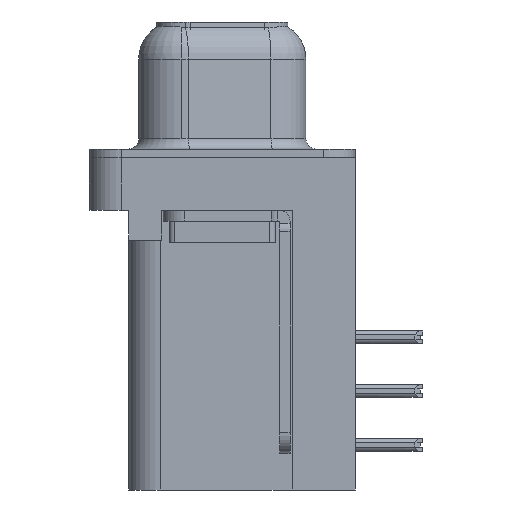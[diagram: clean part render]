
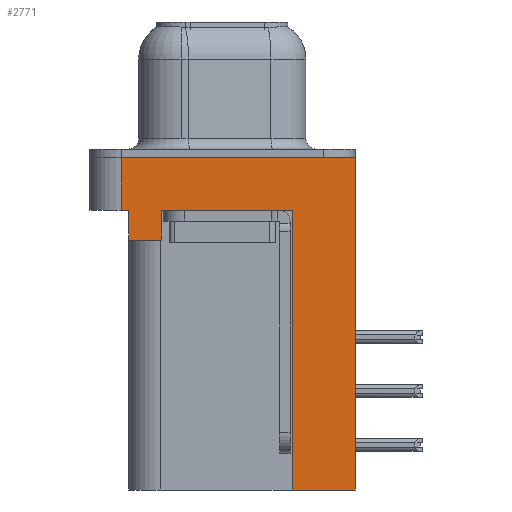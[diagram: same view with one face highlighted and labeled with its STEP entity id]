
A CAD part, left-side view. The second image highlights one B-rep face of the part: STEP entity #2771.
In plain terms, the highlighted planar face has unit normal (-1, 0, 0).
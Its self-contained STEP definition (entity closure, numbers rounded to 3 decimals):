
#1096 = EDGE_CURVE ( 'NONE', #31245, #6564, #27207, .T. ) ;
#1866 = LINE ( 'NONE', #28821, #1961 ) ;
#1961 = VECTOR ( 'NONE', #20287, 1000. ) ;
#2158 = FACE_OUTER_BOUND ( 'NONE', #15014, .T. ) ;
#2771 = ADVANCED_FACE ( 'NONE', ( #2158 ), #19928, .T. ) ;
#3632 = VERTEX_POINT ( 'NONE', #32610 ) ;
#3894 = CARTESIAN_POINT ( 'NONE',  ( -2.935, -6.275, 0. ) ) ;
#6511 = VERTEX_POINT ( 'NONE', #27391 ) ;
#6564 = VERTEX_POINT ( 'NONE', #19073 ) ;
#6860 = VERTEX_POINT ( 'NONE', #9799 ) ;
#7109 = DIRECTION ( 'NONE',  ( 0., 0., 1. ) ) ;
#7168 = ORIENTED_EDGE ( 'NONE', *, *, #12421, .T. ) ;
#7468 = DIRECTION ( 'NONE',  ( 0., -1., 0. ) ) ;
#7547 = VERTEX_POINT ( 'NONE', #25206 ) ;
#8187 = EDGE_CURVE ( 'NONE', #27792, #27473, #30651, .T. ) ;
#9799 = CARTESIAN_POINT ( 'NONE',  ( -2.935, 2.895, -2.5 ) ) ;
#10481 = VECTOR ( 'NONE', #7468, 1000. ) ;
#10658 = CARTESIAN_POINT ( 'NONE',  ( -2.935, 4.775, -2.5 ) ) ;
#10858 = LINE ( 'NONE', #24456, #10481 ) ;
#12023 = CARTESIAN_POINT ( 'NONE',  ( -2.935, 4.425, -3.9 ) ) ;
#12200 = AXIS2_PLACEMENT_3D ( 'NONE', #33886, #17376, #31863 ) ;
#12421 = EDGE_CURVE ( 'NONE', #14638, #6860, #34932, .T. ) ;
#13318 = CARTESIAN_POINT ( 'NONE',  ( -2.935, -6.275, -15.7 ) ) ;
#13356 = EDGE_CURVE ( 'NONE', #6860, #27473, #26138, .T. ) ;
#13749 = VECTOR ( 'NONE', #31548, 1000. ) ;
#13810 = ORIENTED_EDGE ( 'NONE', *, *, #18793, .F. ) ;
#13987 = LINE ( 'NONE', #14246, #13749 ) ;
#14246 = CARTESIAN_POINT ( 'NONE',  ( -2.935, -3.295, -15.7 ) ) ;
#14638 = VERTEX_POINT ( 'NONE', #14997 ) ;
#14676 = DIRECTION ( 'NONE',  ( 0., -1., 0. ) ) ;
#14997 = CARTESIAN_POINT ( 'NONE',  ( -2.935, 2.895, -3.9 ) ) ;
#15014 = EDGE_LOOP ( 'NONE', ( #13810, #24238, #24344, #28443, #22585, #7168, #15855, #29841, #32659, #26134 ) ) ;
#15251 = EDGE_CURVE ( 'NONE', #30735, #7547, #10858, .T. ) ;
#15855 = ORIENTED_EDGE ( 'NONE', *, *, #13356, .T. ) ;
#16312 = EDGE_CURVE ( 'NONE', #14638, #6511, #1866, .T. ) ;
#16382 = CARTESIAN_POINT ( 'NONE',  ( -2.935, -3.295, -15.7 ) ) ;
#16570 = LINE ( 'NONE', #3894, #16882 ) ;
#16882 = VECTOR ( 'NONE', #23689, 1000. ) ;
#16963 = CARTESIAN_POINT ( 'NONE',  ( -2.935, -6.275, -2.5 ) ) ;
#17376 = DIRECTION ( 'NONE',  ( -1., 0., 0. ) ) ;
#17665 = CARTESIAN_POINT ( 'NONE',  ( -2.935, -3.295, -2.5 ) ) ;
#17776 = DIRECTION ( 'NONE',  ( 0., 0., 1. ) ) ;
#18793 = EDGE_CURVE ( 'NONE', #3632, #6564, #16570, .T. ) ;
#19073 = CARTESIAN_POINT ( 'NONE',  ( -2.935, -6.275, 0. ) ) ;
#19217 = EDGE_CURVE ( 'NONE', #31245, #27792, #13987, .T. ) ;
#19928 = PLANE ( 'NONE',  #12200 ) ;
#20287 = DIRECTION ( 'NONE',  ( 0., 1., 0. ) ) ;
#21253 = LINE ( 'NONE', #25036, #21358 ) ;
#21358 = VECTOR ( 'NONE', #27886, 1000. ) ;
#22585 = ORIENTED_EDGE ( 'NONE', *, *, #16312, .F. ) ;
#23689 = DIRECTION ( 'NONE',  ( 0., -1., 0. ) ) ;
#24238 = ORIENTED_EDGE ( 'NONE', *, *, #27805, .F. ) ;
#24344 = ORIENTED_EDGE ( 'NONE', *, *, #15251, .T. ) ;
#24456 = CARTESIAN_POINT ( 'NONE',  ( -2.935, -6.275, -2.5 ) ) ;
#25036 = CARTESIAN_POINT ( 'NONE',  ( -2.935, 4.775, -2.5 ) ) ;
#25206 = CARTESIAN_POINT ( 'NONE',  ( -2.935, 4.425, -2.5 ) ) ;
#25373 = DIRECTION ( 'NONE',  ( 0., 0., 1. ) ) ;
#26134 = ORIENTED_EDGE ( 'NONE', *, *, #1096, .T. ) ;
#26138 = LINE ( 'NONE', #34629, #26641 ) ;
#26234 = EDGE_CURVE ( 'NONE', #6511, #7547, #30275, .T. ) ;
#26641 = VECTOR ( 'NONE', #14676, 1000. ) ;
#26901 = CARTESIAN_POINT ( 'NONE',  ( -2.935, -3.295, -15.7 ) ) ;
#27207 = LINE ( 'NONE', #16963, #28726 ) ;
#27391 = CARTESIAN_POINT ( 'NONE',  ( -2.935, 4.425, -3.9 ) ) ;
#27473 = VERTEX_POINT ( 'NONE', #17665 ) ;
#27792 = VERTEX_POINT ( 'NONE', #16382 ) ;
#27805 = EDGE_CURVE ( 'NONE', #30735, #3632, #21253, .T. ) ;
#27886 = DIRECTION ( 'NONE',  ( 0., 0., 1. ) ) ;
#28443 = ORIENTED_EDGE ( 'NONE', *, *, #26234, .F. ) ;
#28726 = VECTOR ( 'NONE', #25373, 1000. ) ;
#28821 = CARTESIAN_POINT ( 'NONE',  ( -2.935, 4.425, -3.9 ) ) ;
#29756 = VECTOR ( 'NONE', #7109, 1000. ) ;
#29841 = ORIENTED_EDGE ( 'NONE', *, *, #8187, .F. ) ;
#30250 = VECTOR ( 'NONE', #17776, 1000. ) ;
#30275 = LINE ( 'NONE', #12023, #30250 ) ;
#30651 = LINE ( 'NONE', #26901, #29756 ) ;
#30735 = VERTEX_POINT ( 'NONE', #10658 ) ;
#31245 = VERTEX_POINT ( 'NONE', #13318 ) ;
#31548 = DIRECTION ( 'NONE',  ( 0., 1., 0. ) ) ;
#31863 = DIRECTION ( 'NONE',  ( 0., 0., 1. ) ) ;
#32610 = CARTESIAN_POINT ( 'NONE',  ( -2.935, 4.775, 0. ) ) ;
#32659 = ORIENTED_EDGE ( 'NONE', *, *, #19217, .F. ) ;
#32759 = CARTESIAN_POINT ( 'NONE',  ( -2.935, 2.895, -3.9 ) ) ;
#33886 = CARTESIAN_POINT ( 'NONE',  ( -2.935, -6.275, -2.5 ) ) ;
#34629 = CARTESIAN_POINT ( 'NONE',  ( -2.935, -6.275, -2.5 ) ) ;
#34672 = VECTOR ( 'NONE', #35509, 1000. ) ;
#34932 = LINE ( 'NONE', #32759, #34672 ) ;
#35509 = DIRECTION ( 'NONE',  ( 0., 0., 1. ) ) ;
